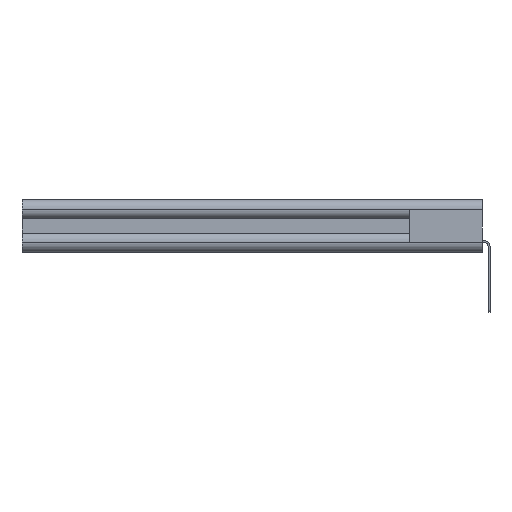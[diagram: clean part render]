
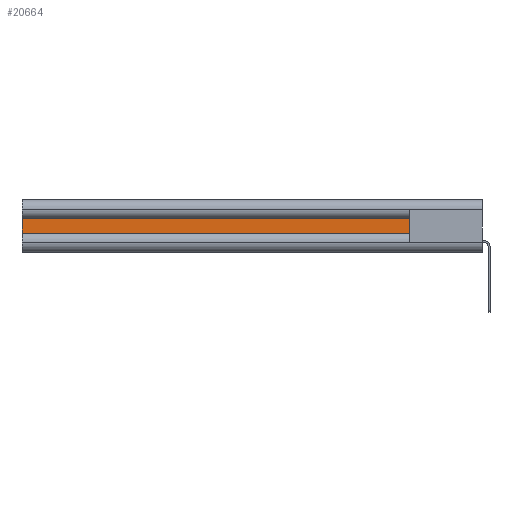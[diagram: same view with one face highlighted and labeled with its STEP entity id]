
A CAD part, left-side view. The second image highlights one B-rep face of the part: STEP entity #20664.
In plain terms, the highlighted planar face has unit normal (-1, 0, 0).
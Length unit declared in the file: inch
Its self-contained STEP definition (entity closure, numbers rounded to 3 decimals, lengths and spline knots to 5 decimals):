
#554 = CARTESIAN_POINT ( 'NONE',  ( 0.044, 3., -0.0465 ) ) ;
#886 = LINE ( 'NONE', #554, #10282 ) ;
#1566 = CARTESIAN_POINT ( 'NONE',  ( 0.044, 3., 0.0465 ) ) ;
#1615 = VERTEX_POINT ( 'NONE', #3070 ) ;
#2467 = DIRECTION ( 'NONE',  ( 0., 0., -1. ) ) ;
#2502 = EDGE_LOOP ( 'NONE', ( #6788, #16445, #16692, #19712 ) ) ;
#3070 = CARTESIAN_POINT ( 'NONE',  ( 0.044, 3., -0.0465 ) ) ;
#3134 = EDGE_CURVE ( 'NONE', #6511, #1615, #13936, .T. ) ;
#3635 = DIRECTION ( 'NONE',  ( 0., 0., -1. ) ) ;
#4215 = VECTOR ( 'NONE', #10585, 39.37008 ) ;
#5011 = AXIS2_PLACEMENT_3D ( 'NONE', #19829, #14574, #3635 ) ;
#6036 = VECTOR ( 'NONE', #15437, 39.37008 ) ;
#6044 = EDGE_CURVE ( 'NONE', #19188, #6511, #7895, .T. ) ;
#6134 = CARTESIAN_POINT ( 'NONE',  ( 0.044, 0.473, -0.0465 ) ) ;
#6511 = VERTEX_POINT ( 'NONE', #6134 ) ;
#6605 = LINE ( 'NONE', #12009, #6036 ) ;
#6788 = ORIENTED_EDGE ( 'NONE', *, *, #21540, .T. ) ;
#7895 = LINE ( 'NONE', #8514, #22045 ) ;
#8514 = CARTESIAN_POINT ( 'NONE',  ( 0.044, 0.473, -0.0465 ) ) ;
#9193 = PLANE ( 'NONE',  #5011 ) ;
#10282 = VECTOR ( 'NONE', #2467, 39.37008 ) ;
#10358 = DIRECTION ( 'NONE',  ( 0., 0., -1. ) ) ;
#10585 = DIRECTION ( 'NONE',  ( 0., 1., 0. ) ) ;
#11429 = CARTESIAN_POINT ( 'NONE',  ( 0.044, 0.37012, -0.0465 ) ) ;
#12009 = CARTESIAN_POINT ( 'NONE',  ( 0.044, 0.37012, 0.0465 ) ) ;
#12224 = CARTESIAN_POINT ( 'NONE',  ( 0.044, 0.473, 0.0465 ) ) ;
#13936 = LINE ( 'NONE', #11429, #4215 ) ;
#14126 = VERTEX_POINT ( 'NONE', #1566 ) ;
#14574 = DIRECTION ( 'NONE',  ( 1., 0., 0. ) ) ;
#15437 = DIRECTION ( 'NONE',  ( 0., 1., 0. ) ) ;
#16445 = ORIENTED_EDGE ( 'NONE', *, *, #18155, .T. ) ;
#16692 = ORIENTED_EDGE ( 'NONE', *, *, #3134, .F. ) ;
#18155 = EDGE_CURVE ( 'NONE', #14126, #1615, #886, .T. ) ;
#18480 = FACE_OUTER_BOUND ( 'NONE', #2502, .T. ) ;
#19188 = VERTEX_POINT ( 'NONE', #12224 ) ;
#19712 = ORIENTED_EDGE ( 'NONE', *, *, #6044, .F. ) ;
#19829 = CARTESIAN_POINT ( 'NONE',  ( 0.044, 0.37012, -0.0465 ) ) ;
#20664 = ADVANCED_FACE ( 'NONE', ( #18480 ), #9193, .F. ) ;
#21540 = EDGE_CURVE ( 'NONE', #19188, #14126, #6605, .T. ) ;
#22045 = VECTOR ( 'NONE', #10358, 39.37008 ) ;
